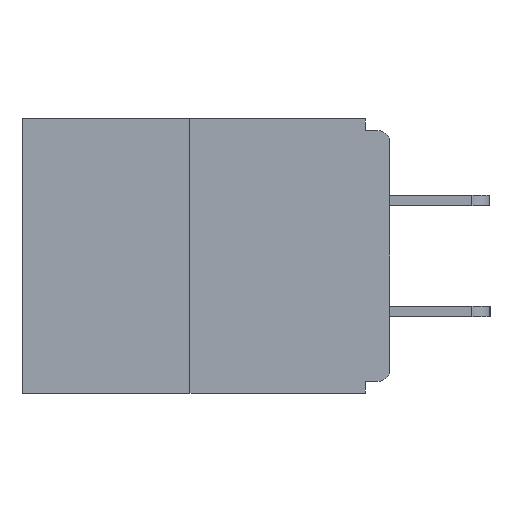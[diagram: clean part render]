
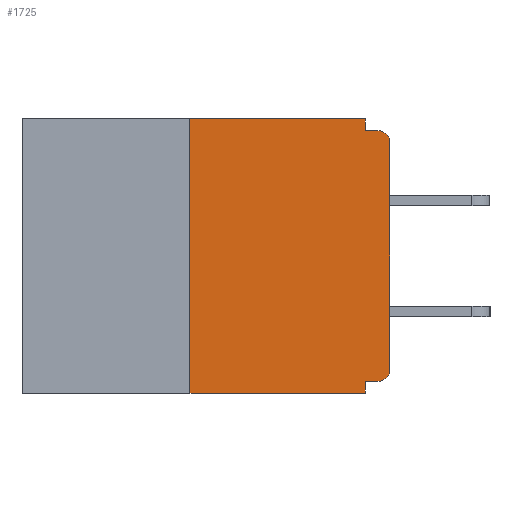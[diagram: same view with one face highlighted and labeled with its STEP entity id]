
A CAD part, left-side view. The second image highlights one B-rep face of the part: STEP entity #1725.
In plain terms, the highlighted planar face has unit normal (-1, 0, 0).
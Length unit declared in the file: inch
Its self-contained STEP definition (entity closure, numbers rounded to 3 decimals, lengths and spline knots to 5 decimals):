
#36 = ORIENTED_EDGE ( 'NONE', *, *, #4295, .F. ) ;
#704 = LINE ( 'NONE', #25585, #2638 ) ;
#712 = ORIENTED_EDGE ( 'NONE', *, *, #17743, .T. ) ;
#878 = VERTEX_POINT ( 'NONE', #13628 ) ;
#909 = EDGE_CURVE ( 'NONE', #878, #2531, #4118, .T. ) ;
#1352 = ORIENTED_EDGE ( 'NONE', *, *, #15722, .T. ) ;
#1725 = ADVANCED_FACE ( 'NONE', ( #7386 ), #9143, .F. ) ;
#1803 = LINE ( 'NONE', #24395, #16928 ) ;
#2446 = LINE ( 'NONE', #14713, #13564 ) ;
#2531 = VERTEX_POINT ( 'NONE', #23476 ) ;
#2638 = VECTOR ( 'NONE', #7164, 39.37008 ) ;
#2962 = VERTEX_POINT ( 'NONE', #26430 ) ;
#3097 = CARTESIAN_POINT ( 'NONE',  ( 0., 0.015, -0.015 ) ) ;
#3315 = CIRCLE ( 'NONE', #24773, 0.015 ) ;
#4118 = LINE ( 'NONE', #13227, #23652 ) ;
#4259 = DIRECTION ( 'NONE',  ( 0., 0., -1. ) ) ;
#4295 = EDGE_CURVE ( 'NONE', #17780, #878, #1803, .T. ) ;
#4705 = VERTEX_POINT ( 'NONE', #20960 ) ;
#6815 = CARTESIAN_POINT ( 'NONE',  ( 0., 0.46, -0.343 ) ) ;
#6979 = EDGE_CURVE ( 'NONE', #19934, #9886, #8359, .T. ) ;
#7142 = CARTESIAN_POINT ( 'NONE',  ( 0., 0.015, -0.328 ) ) ;
#7164 = DIRECTION ( 'NONE',  ( 0., 1., 0. ) ) ;
#7249 = CIRCLE ( 'NONE', #26127, 0.015 ) ;
#7343 = DIRECTION ( 'NONE',  ( 0., 0., 1. ) ) ;
#7386 = FACE_OUTER_BOUND ( 'NONE', #23985, .T. ) ;
#7666 = ORIENTED_EDGE ( 'NONE', *, *, #19916, .T. ) ;
#7707 = ORIENTED_EDGE ( 'NONE', *, *, #16590, .F. ) ;
#7739 = ORIENTED_EDGE ( 'NONE', *, *, #6979, .F. ) ;
#7909 = VECTOR ( 'NONE', #25101, 39.37008 ) ;
#8359 = LINE ( 'NONE', #14706, #24394 ) ;
#9143 = PLANE ( 'NONE',  #13990 ) ;
#9886 = VERTEX_POINT ( 'NONE', #11036 ) ;
#11036 = CARTESIAN_POINT ( 'NONE',  ( 0., 0.031, -0.343 ) ) ;
#12444 = LINE ( 'NONE', #16471, #21162 ) ;
#13227 = CARTESIAN_POINT ( 'NONE',  ( 0., 0.031, 0. ) ) ;
#13564 = VECTOR ( 'NONE', #21004, 39.37008 ) ;
#13604 = ORIENTED_EDGE ( 'NONE', *, *, #909, .F. ) ;
#13628 = CARTESIAN_POINT ( 'NONE',  ( 0., 0.031, 0. ) ) ;
#13990 = AXIS2_PLACEMENT_3D ( 'NONE', #15344, #15604, #23796 ) ;
#14200 = DIRECTION ( 'NONE',  ( 0., -1., 0. ) ) ;
#14235 = VERTEX_POINT ( 'NONE', #7142 ) ;
#14706 = CARTESIAN_POINT ( 'NONE',  ( 0., 0.031, -0.343 ) ) ;
#14713 = CARTESIAN_POINT ( 'NONE',  ( 0., 0., -0.015 ) ) ;
#14837 = DIRECTION ( 'NONE',  ( 0., 0., -1. ) ) ;
#15035 = LINE ( 'NONE', #6815, #7909 ) ;
#15344 = CARTESIAN_POINT ( 'NONE',  ( 0., 0.46, 0. ) ) ;
#15604 = DIRECTION ( 'NONE',  ( 1., 0., 0. ) ) ;
#15722 = EDGE_CURVE ( 'NONE', #16380, #9886, #15035, .T. ) ;
#16380 = VERTEX_POINT ( 'NONE', #25849 ) ;
#16471 = CARTESIAN_POINT ( 'NONE',  ( 0., 0., 0. ) ) ;
#16590 = EDGE_CURVE ( 'NONE', #2531, #22494, #2446, .T. ) ;
#16928 = VECTOR ( 'NONE', #14200, 39.37008 ) ;
#17121 = EDGE_CURVE ( 'NONE', #16380, #17780, #25889, .T. ) ;
#17703 = CARTESIAN_POINT ( 'NONE',  ( 0., 0.25, 0. ) ) ;
#17743 = EDGE_CURVE ( 'NONE', #2962, #22494, #3315, .T. ) ;
#17780 = VERTEX_POINT ( 'NONE', #18069 ) ;
#17851 = DIRECTION ( 'NONE',  ( 0., 0., -1. ) ) ;
#18069 = CARTESIAN_POINT ( 'NONE',  ( 0., 0.25, 0. ) ) ;
#18130 = ORIENTED_EDGE ( 'NONE', *, *, #17121, .F. ) ;
#18196 = DIRECTION ( 'NONE',  ( 0., 0., -1. ) ) ;
#19916 = EDGE_CURVE ( 'NONE', #14235, #4705, #7249, .T. ) ;
#19934 = VERTEX_POINT ( 'NONE', #23888 ) ;
#20630 = DIRECTION ( 'NONE',  ( 0., 0., 1. ) ) ;
#20711 = EDGE_CURVE ( 'NONE', #14235, #19934, #704, .T. ) ;
#20960 = CARTESIAN_POINT ( 'NONE',  ( 0., 0., -0.313 ) ) ;
#21004 = DIRECTION ( 'NONE',  ( 0., -1., 0. ) ) ;
#21162 = VECTOR ( 'NONE', #20630, 39.37008 ) ;
#21860 = EDGE_CURVE ( 'NONE', #4705, #2962, #12444, .T. ) ;
#22225 = CARTESIAN_POINT ( 'NONE',  ( 0., 0.015, -0.03 ) ) ;
#22396 = CARTESIAN_POINT ( 'NONE',  ( 0., 0.015, -0.313 ) ) ;
#22494 = VERTEX_POINT ( 'NONE', #3097 ) ;
#23476 = CARTESIAN_POINT ( 'NONE',  ( 0., 0.031, -0.015 ) ) ;
#23652 = VECTOR ( 'NONE', #4259, 39.37008 ) ;
#23796 = DIRECTION ( 'NONE',  ( 0., 0., -1. ) ) ;
#23888 = CARTESIAN_POINT ( 'NONE',  ( 0., 0.031, -0.328 ) ) ;
#23985 = EDGE_LOOP ( 'NONE', ( #36, #18130, #1352, #7739, #24945, #7666, #24263, #712, #7707, #13604 ) ) ;
#24263 = ORIENTED_EDGE ( 'NONE', *, *, #21860, .T. ) ;
#24394 = VECTOR ( 'NONE', #14837, 39.37008 ) ;
#24395 = CARTESIAN_POINT ( 'NONE',  ( 0., 0.46, 0. ) ) ;
#24509 = DIRECTION ( 'NONE',  ( -1., 0., 0. ) ) ;
#24773 = AXIS2_PLACEMENT_3D ( 'NONE', #22225, #24509, #18196 ) ;
#24945 = ORIENTED_EDGE ( 'NONE', *, *, #20711, .F. ) ;
#25101 = DIRECTION ( 'NONE',  ( 0., -1., 0. ) ) ;
#25585 = CARTESIAN_POINT ( 'NONE',  ( 0., 0., -0.328 ) ) ;
#25849 = CARTESIAN_POINT ( 'NONE',  ( 0., 0.25, -0.343 ) ) ;
#25889 = LINE ( 'NONE', #17703, #26011 ) ;
#26011 = VECTOR ( 'NONE', #7343, 39.37008 ) ;
#26127 = AXIS2_PLACEMENT_3D ( 'NONE', #22396, #26561, #17851 ) ;
#26430 = CARTESIAN_POINT ( 'NONE',  ( 0., 0., -0.03 ) ) ;
#26561 = DIRECTION ( 'NONE',  ( -1., 0., 0. ) ) ;
